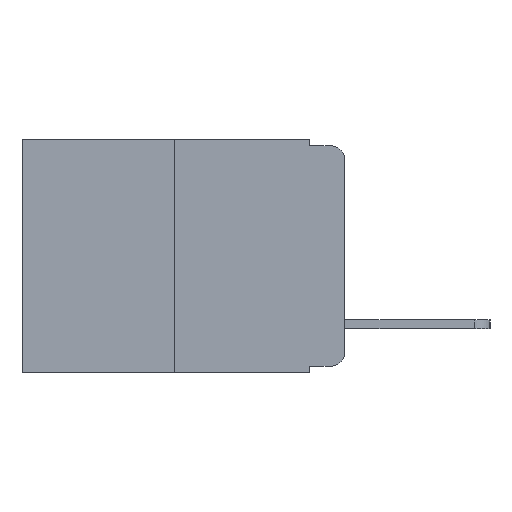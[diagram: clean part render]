
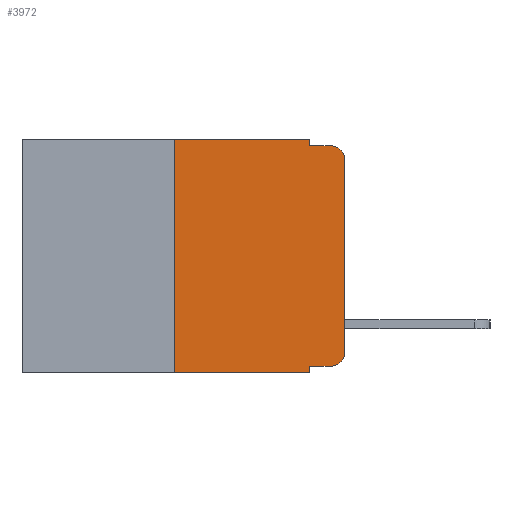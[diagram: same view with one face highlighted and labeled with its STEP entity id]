
A CAD part, left-side view. The second image highlights one B-rep face of the part: STEP entity #3972.
In plain terms, the highlighted planar face has unit normal (-1, 0, 0).
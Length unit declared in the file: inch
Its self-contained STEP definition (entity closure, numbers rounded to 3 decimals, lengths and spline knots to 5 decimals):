
#127 = VECTOR ( 'NONE', #6034, 39.37008 ) ;
#239 = CARTESIAN_POINT ( 'NONE',  ( 0., 0.02, -0.03 ) ) ;
#384 = ORIENTED_EDGE ( 'NONE', *, *, #23542, .T. ) ;
#533 = CARTESIAN_POINT ( 'NONE',  ( 0., 0.051, -0.01 ) ) ;
#893 = DIRECTION ( 'NONE',  ( 0., -1., 0. ) ) ;
#1000 = VERTEX_POINT ( 'NONE', #3262 ) ;
#1008 = DIRECTION ( 'NONE',  ( 0., 0., -1. ) ) ;
#1075 = EDGE_CURVE ( 'NONE', #18357, #21515, #22737, .T. ) ;
#1107 = VECTOR ( 'NONE', #8382, 39.37008 ) ;
#1404 = LINE ( 'NONE', #533, #20280 ) ;
#1646 = DIRECTION ( 'NONE',  ( 0., -1., 0. ) ) ;
#1767 = AXIS2_PLACEMENT_3D ( 'NONE', #2261, #15146, #4193 ) ;
#1823 = VERTEX_POINT ( 'NONE', #15496 ) ;
#2139 = DIRECTION ( 'NONE',  ( 0., 0., -1. ) ) ;
#2261 = CARTESIAN_POINT ( 'NONE',  ( 0., 0.02, -0.313 ) ) ;
#2512 = DIRECTION ( 'NONE',  ( 0., -1., 0. ) ) ;
#2617 = CARTESIAN_POINT ( 'NONE',  ( 0., 0., -0.03 ) ) ;
#2796 = CARTESIAN_POINT ( 'NONE',  ( 0., 0.473, -0.343 ) ) ;
#3262 = CARTESIAN_POINT ( 'NONE',  ( 0., 0.25, -0.343 ) ) ;
#3551 = ORIENTED_EDGE ( 'NONE', *, *, #9838, .T. ) ;
#3565 = CARTESIAN_POINT ( 'NONE',  ( 0., 0.051, -0.343 ) ) ;
#3608 = EDGE_CURVE ( 'NONE', #1000, #1823, #11396, .T. ) ;
#3705 = AXIS2_PLACEMENT_3D ( 'NONE', #18305, #14759, #3771 ) ;
#3771 = DIRECTION ( 'NONE',  ( 0., 0., -1. ) ) ;
#3824 = LINE ( 'NONE', #12123, #23157 ) ;
#3972 = ADVANCED_FACE ( 'NONE', ( #8820 ), #21895, .F. ) ;
#4193 = DIRECTION ( 'NONE',  ( 0., 0., -1. ) ) ;
#4648 = LINE ( 'NONE', #9094, #23363 ) ;
#4865 = EDGE_CURVE ( 'NONE', #15641, #16425, #3824, .T. ) ;
#5017 = AXIS2_PLACEMENT_3D ( 'NONE', #239, #13195, #2139 ) ;
#5298 = CARTESIAN_POINT ( 'NONE',  ( 0., 0.02, -0.01 ) ) ;
#5431 = VERTEX_POINT ( 'NONE', #2617 ) ;
#6034 = DIRECTION ( 'NONE',  ( 0., 0., 1. ) ) ;
#6165 = ORIENTED_EDGE ( 'NONE', *, *, #1075, .F. ) ;
#6399 = CARTESIAN_POINT ( 'NONE',  ( 0., 0.25, 0. ) ) ;
#6510 = CARTESIAN_POINT ( 'NONE',  ( 0., 0.473, 0. ) ) ;
#6595 = ORIENTED_EDGE ( 'NONE', *, *, #8611, .T. ) ;
#6792 = ORIENTED_EDGE ( 'NONE', *, *, #7351, .F. ) ;
#7351 = EDGE_CURVE ( 'NONE', #16425, #12536, #1404, .T. ) ;
#7571 = EDGE_LOOP ( 'NONE', ( #3551, #6595, #6792, #13508, #17874, #10080, #8221, #6165, #384, #22897 ) ) ;
#7624 = CARTESIAN_POINT ( 'NONE',  ( 0., 0.051, -0.333 ) ) ;
#7925 = CARTESIAN_POINT ( 'NONE',  ( 0., 0., -0.313 ) ) ;
#8221 = ORIENTED_EDGE ( 'NONE', *, *, #19348, .T. ) ;
#8269 = DIRECTION ( 'NONE',  ( 0., 0., 1. ) ) ;
#8382 = DIRECTION ( 'NONE',  ( 0., -1., 0. ) ) ;
#8491 = CIRCLE ( 'NONE', #1767, 0.02 ) ;
#8611 = EDGE_CURVE ( 'NONE', #5431, #12536, #17181, .T. ) ;
#8820 = FACE_OUTER_BOUND ( 'NONE', #7571, .T. ) ;
#9094 = CARTESIAN_POINT ( 'NONE',  ( 0., 0.051, -0.333 ) ) ;
#9838 = EDGE_CURVE ( 'NONE', #11070, #5431, #10089, .T. ) ;
#10080 = ORIENTED_EDGE ( 'NONE', *, *, #3608, .F. ) ;
#10089 = LINE ( 'NONE', #18739, #127 ) ;
#10439 = CARTESIAN_POINT ( 'NONE',  ( 0., 0.051, -0.01 ) ) ;
#11070 = VERTEX_POINT ( 'NONE', #7925 ) ;
#11396 = LINE ( 'NONE', #6399, #20974 ) ;
#12123 = CARTESIAN_POINT ( 'NONE',  ( 0., 0.051, 0. ) ) ;
#12536 = VERTEX_POINT ( 'NONE', #5298 ) ;
#13195 = DIRECTION ( 'NONE',  ( -1., 0., 0. ) ) ;
#13375 = VECTOR ( 'NONE', #893, 39.37008 ) ;
#13508 = ORIENTED_EDGE ( 'NONE', *, *, #4865, .F. ) ;
#13810 = VERTEX_POINT ( 'NONE', #20307 ) ;
#14321 = DIRECTION ( 'NONE',  ( 0., 0., -1. ) ) ;
#14412 = CARTESIAN_POINT ( 'NONE',  ( 0., 0.051, 0. ) ) ;
#14759 = DIRECTION ( 'NONE',  ( 1., 0., 0. ) ) ;
#15146 = DIRECTION ( 'NONE',  ( -1., 0., 0. ) ) ;
#15496 = CARTESIAN_POINT ( 'NONE',  ( 0., 0.25, 0. ) ) ;
#15590 = CARTESIAN_POINT ( 'NONE',  ( 0., 0.051, 0. ) ) ;
#15641 = VERTEX_POINT ( 'NONE', #15590 ) ;
#15818 = LINE ( 'NONE', #6510, #1107 ) ;
#16425 = VERTEX_POINT ( 'NONE', #10439 ) ;
#17181 = CIRCLE ( 'NONE', #5017, 0.02 ) ;
#17874 = ORIENTED_EDGE ( 'NONE', *, *, #23282, .F. ) ;
#18305 = CARTESIAN_POINT ( 'NONE',  ( 0., 0.473, 0. ) ) ;
#18357 = VERTEX_POINT ( 'NONE', #7624 ) ;
#18515 = VECTOR ( 'NONE', #14321, 39.37008 ) ;
#18739 = CARTESIAN_POINT ( 'NONE',  ( 0., 0., 0. ) ) ;
#19348 = EDGE_CURVE ( 'NONE', #1000, #21515, #22961, .T. ) ;
#20280 = VECTOR ( 'NONE', #2512, 39.37008 ) ;
#20307 = CARTESIAN_POINT ( 'NONE',  ( 0., 0.02, -0.333 ) ) ;
#20974 = VECTOR ( 'NONE', #8269, 39.37008 ) ;
#21515 = VERTEX_POINT ( 'NONE', #3565 ) ;
#21895 = PLANE ( 'NONE',  #3705 ) ;
#22337 = EDGE_CURVE ( 'NONE', #13810, #11070, #8491, .T. ) ;
#22737 = LINE ( 'NONE', #14412, #18515 ) ;
#22897 = ORIENTED_EDGE ( 'NONE', *, *, #22337, .T. ) ;
#22961 = LINE ( 'NONE', #2796, #13375 ) ;
#23157 = VECTOR ( 'NONE', #1008, 39.37008 ) ;
#23282 = EDGE_CURVE ( 'NONE', #1823, #15641, #15818, .T. ) ;
#23363 = VECTOR ( 'NONE', #1646, 39.37008 ) ;
#23542 = EDGE_CURVE ( 'NONE', #18357, #13810, #4648, .T. ) ;
